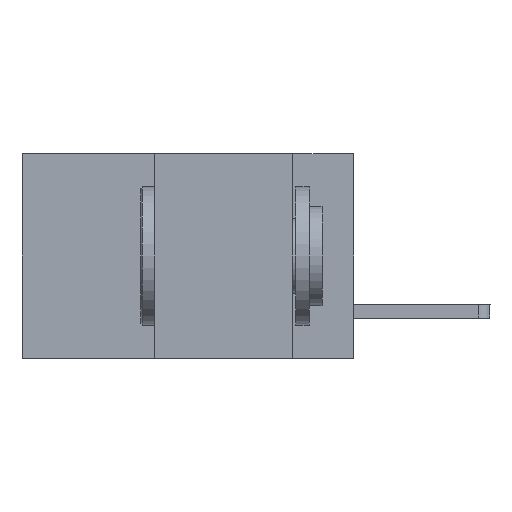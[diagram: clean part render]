
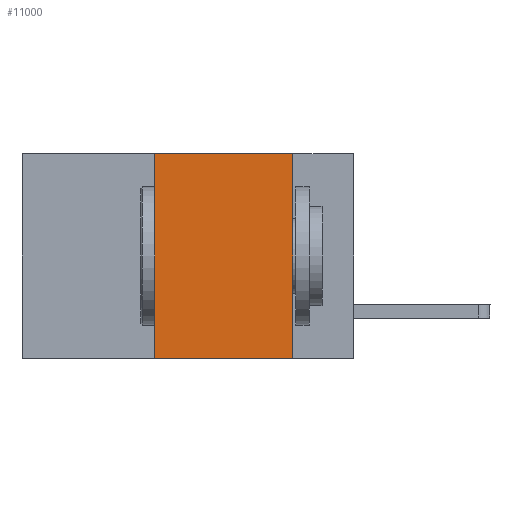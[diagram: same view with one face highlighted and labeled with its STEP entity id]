
A CAD part, left-side view. The second image highlights one B-rep face of the part: STEP entity #11000.
In plain terms, the highlighted planar face has unit normal (-1, 0, 0).
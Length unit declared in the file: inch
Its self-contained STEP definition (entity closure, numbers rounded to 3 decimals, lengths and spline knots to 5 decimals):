
#457 = CARTESIAN_POINT ( 'NONE',  ( 0., 0.6, 0. ) ) ;
#502 = EDGE_CURVE ( 'NONE', #1169, #7714, #9068, .T. ) ;
#599 = CARTESIAN_POINT ( 'NONE',  ( 0., 0.36, -0.37 ) ) ;
#756 = VECTOR ( 'NONE', #1995, 39.37008 ) ;
#1169 = VERTEX_POINT ( 'NONE', #599 ) ;
#1292 = CARTESIAN_POINT ( 'NONE',  ( 0., 0.36, 0. ) ) ;
#1995 = DIRECTION ( 'NONE',  ( 0., -1., 0. ) ) ;
#2185 = CARTESIAN_POINT ( 'NONE',  ( 0., 0.11, 0. ) ) ;
#2791 = EDGE_CURVE ( 'NONE', #7005, #7714, #4736, .T. ) ;
#3154 = ORIENTED_EDGE ( 'NONE', *, *, #2791, .F. ) ;
#3216 = DIRECTION ( 'NONE',  ( 0., 0., -1. ) ) ;
#4014 = ORIENTED_EDGE ( 'NONE', *, *, #8900, .F. ) ;
#4166 = DIRECTION ( 'NONE',  ( 0., 0., 1. ) ) ;
#4736 = LINE ( 'NONE', #7660, #9001 ) ;
#4743 = EDGE_CURVE ( 'NONE', #5780, #7005, #6785, .T. ) ;
#5032 = ORIENTED_EDGE ( 'NONE', *, *, #4743, .F. ) ;
#5395 = AXIS2_PLACEMENT_3D ( 'NONE', #9876, #10737, #8212 ) ;
#5557 = CARTESIAN_POINT ( 'NONE',  ( 0., 0.11, -0.37 ) ) ;
#5580 = PLANE ( 'NONE',  #5395 ) ;
#5640 = DIRECTION ( 'NONE',  ( 0., -1., 0. ) ) ;
#5780 = VERTEX_POINT ( 'NONE', #1292 ) ;
#6710 = VECTOR ( 'NONE', #5640, 39.37008 ) ;
#6785 = LINE ( 'NONE', #457, #756 ) ;
#7005 = VERTEX_POINT ( 'NONE', #2185 ) ;
#7123 = LINE ( 'NONE', #7650, #11334 ) ;
#7575 = EDGE_LOOP ( 'NONE', ( #3154, #5032, #4014, #9765 ) ) ;
#7650 = CARTESIAN_POINT ( 'NONE',  ( 0., 0.36, 0. ) ) ;
#7660 = CARTESIAN_POINT ( 'NONE',  ( 0., 0.11, 0. ) ) ;
#7714 = VERTEX_POINT ( 'NONE', #5557 ) ;
#8212 = DIRECTION ( 'NONE',  ( 0., 0., -1. ) ) ;
#8900 = EDGE_CURVE ( 'NONE', #1169, #5780, #7123, .T. ) ;
#8901 = FACE_OUTER_BOUND ( 'NONE', #7575, .T. ) ;
#9001 = VECTOR ( 'NONE', #3216, 39.37008 ) ;
#9068 = LINE ( 'NONE', #9127, #6710 ) ;
#9127 = CARTESIAN_POINT ( 'NONE',  ( 0., 0.6, -0.37 ) ) ;
#9765 = ORIENTED_EDGE ( 'NONE', *, *, #502, .T. ) ;
#9876 = CARTESIAN_POINT ( 'NONE',  ( 0., 0.6, 0. ) ) ;
#10737 = DIRECTION ( 'NONE',  ( 1., 0., 0. ) ) ;
#11000 = ADVANCED_FACE ( 'NONE', ( #8901 ), #5580, .F. ) ;
#11334 = VECTOR ( 'NONE', #4166, 39.37008 ) ;
